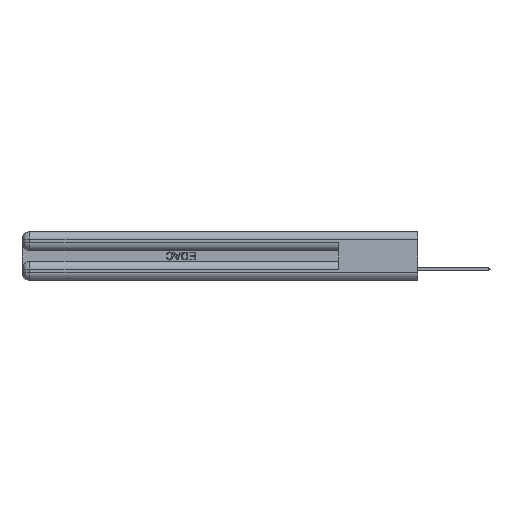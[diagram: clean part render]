
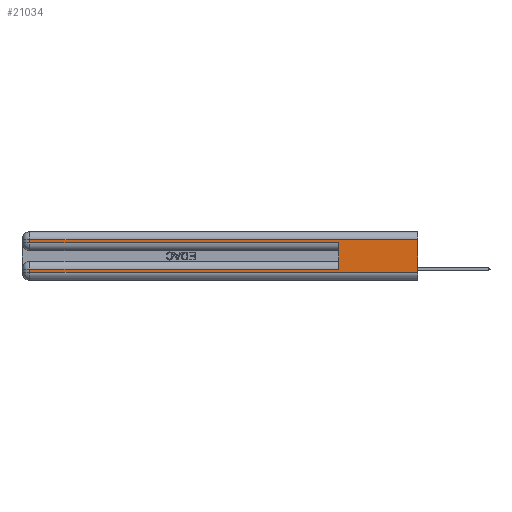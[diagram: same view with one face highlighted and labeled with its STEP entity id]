
A CAD part, left-side view. The second image highlights one B-rep face of the part: STEP entity #21034.
In plain terms, the highlighted planar face has unit normal (-1, 0, 0).
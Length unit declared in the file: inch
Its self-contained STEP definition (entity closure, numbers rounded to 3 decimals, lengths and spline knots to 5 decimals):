
#249 = CARTESIAN_POINT ( 'NONE',  ( 0., 2.94, 0.085 ) ) ;
#656 = CARTESIAN_POINT ( 'NONE',  ( 0., 0.6, 0.285 ) ) ;
#824 = CARTESIAN_POINT ( 'NONE',  ( 0., 2.94, 0.06 ) ) ;
#1630 = CARTESIAN_POINT ( 'NONE',  ( 0., 0., 0.37 ) ) ;
#1746 = DIRECTION ( 'NONE',  ( 0., 1., 0. ) ) ;
#2286 = VERTEX_POINT ( 'NONE', #20897 ) ;
#3185 = VECTOR ( 'NONE', #37701, 39.37008 ) ;
#3481 = ORIENTED_EDGE ( 'NONE', *, *, #5884, .T. ) ;
#4053 = EDGE_CURVE ( 'NONE', #45496, #30306, #29907, .T. ) ;
#4196 = DIRECTION ( 'NONE',  ( 0., 0., 1. ) ) ;
#5050 = DIRECTION ( 'NONE',  ( 0., 0., -1. ) ) ;
#5884 = EDGE_CURVE ( 'NONE', #2286, #8350, #45315, .T. ) ;
#6694 = LINE ( 'NONE', #15209, #3185 ) ;
#6822 = CARTESIAN_POINT ( 'NONE',  ( 0., 0., 0.06 ) ) ;
#7657 = LINE ( 'NONE', #44923, #46969 ) ;
#8350 = VERTEX_POINT ( 'NONE', #249 ) ;
#9399 = ORIENTED_EDGE ( 'NONE', *, *, #15740, .F. ) ;
#9710 = EDGE_CURVE ( 'NONE', #22274, #30306, #22741, .T. ) ;
#11766 = DIRECTION ( 'NONE',  ( 0., 0., -1. ) ) ;
#13455 = DIRECTION ( 'NONE',  ( 0., -1., 0. ) ) ;
#14037 = ORIENTED_EDGE ( 'NONE', *, *, #9710, .F. ) ;
#14125 = LINE ( 'NONE', #23837, #19902 ) ;
#14791 = DIRECTION ( 'NONE',  ( 0., 0., -1. ) ) ;
#14803 = EDGE_CURVE ( 'NONE', #27033, #28422, #14125, .T. ) ;
#15109 = AXIS2_PLACEMENT_3D ( 'NONE', #1630, #20278, #5050 ) ;
#15153 = ORIENTED_EDGE ( 'NONE', *, *, #20605, .T. ) ;
#15209 = CARTESIAN_POINT ( 'NONE',  ( 0., 2.94, 0.37 ) ) ;
#15740 = EDGE_CURVE ( 'NONE', #2286, #28422, #26720, .T. ) ;
#16631 = ORIENTED_EDGE ( 'NONE', *, *, #21746, .T. ) ;
#18942 = CARTESIAN_POINT ( 'NONE',  ( 0., 0., 0.31 ) ) ;
#19074 = ORIENTED_EDGE ( 'NONE', *, *, #14803, .T. ) ;
#19859 = DIRECTION ( 'NONE',  ( 0., 1., 0. ) ) ;
#19902 = VECTOR ( 'NONE', #40956, 39.37008 ) ;
#20049 = VECTOR ( 'NONE', #13455, 39.37008 ) ;
#20278 = DIRECTION ( 'NONE',  ( 1., 0., 0. ) ) ;
#20605 = EDGE_CURVE ( 'NONE', #22274, #29962, #39600, .T. ) ;
#20897 = CARTESIAN_POINT ( 'NONE',  ( 0., 0.6, 0.085 ) ) ;
#21034 = ADVANCED_FACE ( 'NONE', ( #34356 ), #27241, .F. ) ;
#21550 = VECTOR ( 'NONE', #4196, 39.37008 ) ;
#21746 = EDGE_CURVE ( 'NONE', #29962, #27033, #7657, .T. ) ;
#22274 = VERTEX_POINT ( 'NONE', #18942 ) ;
#22741 = LINE ( 'NONE', #29821, #26773 ) ;
#23837 = CARTESIAN_POINT ( 'NONE',  ( 0., 0., 0.285 ) ) ;
#24484 = EDGE_CURVE ( 'NONE', #8350, #45496, #6694, .T. ) ;
#24595 = CARTESIAN_POINT ( 'NONE',  ( 0., 0., 0.06 ) ) ;
#26388 = CARTESIAN_POINT ( 'NONE',  ( 0., 0.6, 0.145 ) ) ;
#26720 = LINE ( 'NONE', #26388, #21550 ) ;
#26773 = VECTOR ( 'NONE', #14791, 39.37008 ) ;
#27033 = VERTEX_POINT ( 'NONE', #47589 ) ;
#27152 = CARTESIAN_POINT ( 'NONE',  ( 0., 0., 0.31 ) ) ;
#27241 = PLANE ( 'NONE',  #15109 ) ;
#28422 = VERTEX_POINT ( 'NONE', #656 ) ;
#28876 = CARTESIAN_POINT ( 'NONE',  ( 0., 0., 0.085 ) ) ;
#29821 = CARTESIAN_POINT ( 'NONE',  ( 0., 0., 0.37 ) ) ;
#29907 = LINE ( 'NONE', #24595, #20049 ) ;
#29962 = VERTEX_POINT ( 'NONE', #31295 ) ;
#30306 = VERTEX_POINT ( 'NONE', #6822 ) ;
#31295 = CARTESIAN_POINT ( 'NONE',  ( 0., 2.94, 0.31 ) ) ;
#33235 = VECTOR ( 'NONE', #19859, 39.37008 ) ;
#34356 = FACE_OUTER_BOUND ( 'NONE', #47682, .T. ) ;
#35544 = VECTOR ( 'NONE', #1746, 39.37008 ) ;
#36955 = ORIENTED_EDGE ( 'NONE', *, *, #4053, .T. ) ;
#37701 = DIRECTION ( 'NONE',  ( 0., 0., -1. ) ) ;
#39600 = LINE ( 'NONE', #27152, #33235 ) ;
#40956 = DIRECTION ( 'NONE',  ( 0., -1., 0. ) ) ;
#42824 = ORIENTED_EDGE ( 'NONE', *, *, #24484, .T. ) ;
#44923 = CARTESIAN_POINT ( 'NONE',  ( 0., 2.94, 0.37 ) ) ;
#45315 = LINE ( 'NONE', #28876, #35544 ) ;
#45496 = VERTEX_POINT ( 'NONE', #824 ) ;
#46969 = VECTOR ( 'NONE', #11766, 39.37008 ) ;
#47589 = CARTESIAN_POINT ( 'NONE',  ( 0., 2.94, 0.285 ) ) ;
#47682 = EDGE_LOOP ( 'NONE', ( #14037, #15153, #16631, #19074, #9399, #3481, #42824, #36955 ) ) ;
